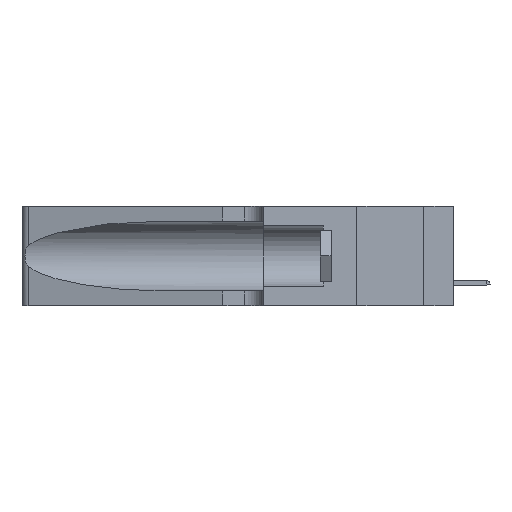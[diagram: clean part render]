
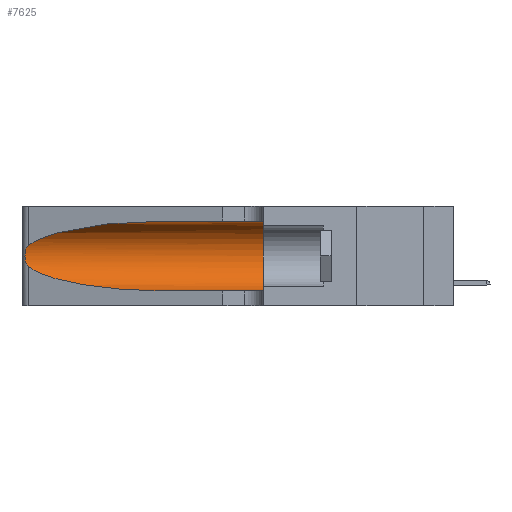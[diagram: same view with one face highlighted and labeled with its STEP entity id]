
A CAD part, left-side view. The second image highlights one B-rep face of the part: STEP entity #7625.
In plain terms, the highlighted cylindrical face has radius 3.308 mm (diameter 6.617 mm), a partial arc.
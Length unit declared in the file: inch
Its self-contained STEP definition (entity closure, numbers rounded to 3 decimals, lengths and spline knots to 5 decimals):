
#74 = CARTESIAN_POINT ( 'NONE',  ( 0.1305, 0.72297, 0.05475 ) ) ;
#592 = CARTESIAN_POINT ( 'NONE',  ( 0.25487, 1.22718, 0.22369 ) ) ;
#1490 = CARTESIAN_POINT ( 'NONE',  ( 0.25856, 1.23593, 0.16098 ) ) ;
#1722 = CARTESIAN_POINT ( 'NONE',  ( 0.25787, 1.23484, 0.2124 ) ) ;
#2198 = CARTESIAN_POINT ( 'NONE',  ( 0.26075, 1.23896, 0.178 ) ) ;
#3631 = ORIENTED_EDGE ( 'NONE', *, *, #31548, .F. ) ;
#4549 = EDGE_CURVE ( 'NONE', #17791, #12352, #44932, .T. ) ;
#4906 = EDGE_CURVE ( 'NONE', #17791, #6363, #7451, .T. ) ;
#4997 = DIRECTION ( 'NONE',  ( 0., -1., 0. ) ) ;
#6036 = DIRECTION ( 'NONE',  ( 0., -1., 0. ) ) ;
#6122 = ORIENTED_EDGE ( 'NONE', *, *, #45249, .T. ) ;
#6363 = VERTEX_POINT ( 'NONE', #44007 ) ;
#6792 = DIRECTION ( 'NONE',  ( 0., 1., 0. ) ) ;
#7451 =( BOUNDED_CURVE ( )  B_SPLINE_CURVE ( 3, ( #11649, #14323, #36444, #592 ),
 .UNSPECIFIED., .F., .F. ) 
 B_SPLINE_CURVE_WITH_KNOTS ( ( 4, 4 ),
 ( 1.5708, 2.84003 ),
 .UNSPECIFIED. ) 
 CURVE ( )  GEOMETRIC_REPRESENTATION_ITEM ( )  RATIONAL_B_SPLINE_CURVE ( ( 1., 0.87, 0.87, 1. ) ) 
 REPRESENTATION_ITEM ( '' )  );
#7625 = ADVANCED_FACE ( 'NONE', ( #20160 ), #38208, .F. ) ;
#7801 = CARTESIAN_POINT ( 'NONE',  ( 0.2373, 1.15595, 0.08982 ) ) ;
#8704 = CARTESIAN_POINT ( 'NONE',  ( 0.25487, 1.22718, 0.14631 ) ) ;
#8941 = CARTESIAN_POINT ( 'NONE',  ( 0.25555, 1.22994, 0.2215 ) ) ;
#9288 =( BOUNDED_CURVE ( )  B_SPLINE_CURVE ( 3, ( #44394, #7801, #15037, #33543 ),
 .UNSPECIFIED., .F., .F. ) 
 B_SPLINE_CURVE_WITH_KNOTS ( ( 4, 4 ),
 ( 3.44316, 4.71239 ),
 .UNSPECIFIED. ) 
 CURVE ( )  GEOMETRIC_REPRESENTATION_ITEM ( )  RATIONAL_B_SPLINE_CURVE ( ( 1., 0.87, 0.87, 1. ) ) 
 REPRESENTATION_ITEM ( '' )  );
#9412 = CARTESIAN_POINT ( 'NONE',  ( 0.25487, 1.22718, 0.22369 ) ) ;
#9653 = CARTESIAN_POINT ( 'NONE',  ( 0.1305, 1.61858, 0.05475 ) ) ;
#11649 = CARTESIAN_POINT ( 'NONE',  ( 0.1305, 0.72297, 0.31525 ) ) ;
#11990 = DIRECTION ( 'NONE',  ( 0., 0., -1. ) ) ;
#12352 = VERTEX_POINT ( 'NONE', #21172 ) ;
#12964 = CARTESIAN_POINT ( 'NONE',  ( 0.1305, 0.72297, 0.31525 ) ) ;
#14323 = CARTESIAN_POINT ( 'NONE',  ( 0.18966, 0.96281, 0.31525 ) ) ;
#14932 = VERTEX_POINT ( 'NONE', #44869 ) ;
#15037 = CARTESIAN_POINT ( 'NONE',  ( 0.18966, 0.96281, 0.05475 ) ) ;
#16129 = EDGE_CURVE ( 'NONE', #27680, #30005, #9288, .T. ) ;
#16179 = CARTESIAN_POINT ( 'NONE',  ( 0.25639, 1.23186, 0.15144 ) ) ;
#17590 = ORIENTED_EDGE ( 'NONE', *, *, #4906, .T. ) ;
#17791 = VERTEX_POINT ( 'NONE', #12964 ) ;
#20160 = FACE_OUTER_BOUND ( 'NONE', #32192, .T. ) ;
#20484 = CARTESIAN_POINT ( 'NONE',  ( 0.25854, 1.2359, 0.20912 ) ) ;
#21172 = CARTESIAN_POINT ( 'NONE',  ( 0.1305, 0.35, 0.31525 ) ) ;
#21948 = DIRECTION ( 'NONE',  ( 0., 0., 1. ) ) ;
#23191 = EDGE_CURVE ( 'NONE', #30005, #14932, #42867, .T. ) ;
#23683 = AXIS2_PLACEMENT_3D ( 'NONE', #47240, #6792, #21948 ) ;
#25435 = DIRECTION ( 'NONE',  ( 0., -1., 0. ) ) ;
#25515 = VECTOR ( 'NONE', #25435, 39.37008 ) ;
#27124 = B_SPLINE_CURVE_WITH_KNOTS ( 'NONE', 3,
 ( #9412, #8941, #38525, #1722, #20484, #41677, #35149, #2198, #39004, #1490, #34663, #16179, #27472, #8704 ),
 .UNSPECIFIED., .F., .F.,
 ( 4, 2, 2, 2, 2, 2, 4 ),
 ( 0., 0.00027, 0.00053, 0.00107, 0.0016, 0.00187, 0.00214 ),
 .UNSPECIFIED. ) ;
#27472 = CARTESIAN_POINT ( 'NONE',  ( 0.25555, 1.22993, 0.14849 ) ) ;
#27680 = VERTEX_POINT ( 'NONE', #46652 ) ;
#28493 = ORIENTED_EDGE ( 'NONE', *, *, #16129, .T. ) ;
#29559 = AXIS2_PLACEMENT_3D ( 'NONE', #34105, #4997, #11990 ) ;
#30005 = VERTEX_POINT ( 'NONE', #74 ) ;
#30595 = CIRCLE ( 'NONE', #23683, 0.13025 ) ;
#31548 = EDGE_CURVE ( 'NONE', #12352, #14932, #30595, .T. ) ;
#32192 = EDGE_LOOP ( 'NONE', ( #17590, #6122, #28493, #35299, #3631, #42336 ) ) ;
#33543 = CARTESIAN_POINT ( 'NONE',  ( 0.1305, 0.72297, 0.05475 ) ) ;
#34105 = CARTESIAN_POINT ( 'NONE',  ( 0.1305, 1.61858, 0.185 ) ) ;
#34663 = CARTESIAN_POINT ( 'NONE',  ( 0.25789, 1.23486, 0.15765 ) ) ;
#35149 = CARTESIAN_POINT ( 'NONE',  ( 0.26075, 1.23896, 0.19203 ) ) ;
#35299 = ORIENTED_EDGE ( 'NONE', *, *, #23191, .T. ) ;
#36444 = CARTESIAN_POINT ( 'NONE',  ( 0.2373, 1.15595, 0.28018 ) ) ;
#38208 = CYLINDRICAL_SURFACE ( 'NONE', #29559, 0.13025 ) ;
#38525 = CARTESIAN_POINT ( 'NONE',  ( 0.25639, 1.23184, 0.21858 ) ) ;
#39004 = CARTESIAN_POINT ( 'NONE',  ( 0.26017, 1.23833, 0.17102 ) ) ;
#41677 = CARTESIAN_POINT ( 'NONE',  ( 0.26018, 1.23835, 0.19895 ) ) ;
#42336 = ORIENTED_EDGE ( 'NONE', *, *, #4549, .F. ) ;
#42867 = LINE ( 'NONE', #9653, #43793 ) ;
#43793 = VECTOR ( 'NONE', #6036, 39.37008 ) ;
#44007 = CARTESIAN_POINT ( 'NONE',  ( 0.25487, 1.22718, 0.22369 ) ) ;
#44206 = CARTESIAN_POINT ( 'NONE',  ( 0.1305, 1.61858, 0.31525 ) ) ;
#44394 = CARTESIAN_POINT ( 'NONE',  ( 0.25487, 1.22718, 0.14631 ) ) ;
#44869 = CARTESIAN_POINT ( 'NONE',  ( 0.1305, 0.35, 0.05475 ) ) ;
#44932 = LINE ( 'NONE', #44206, #25515 ) ;
#45249 = EDGE_CURVE ( 'NONE', #6363, #27680, #27124, .T. ) ;
#46652 = CARTESIAN_POINT ( 'NONE',  ( 0.25487, 1.22718, 0.14631 ) ) ;
#47240 = CARTESIAN_POINT ( 'NONE',  ( 0.1305, 0.35, 0.185 ) ) ;
